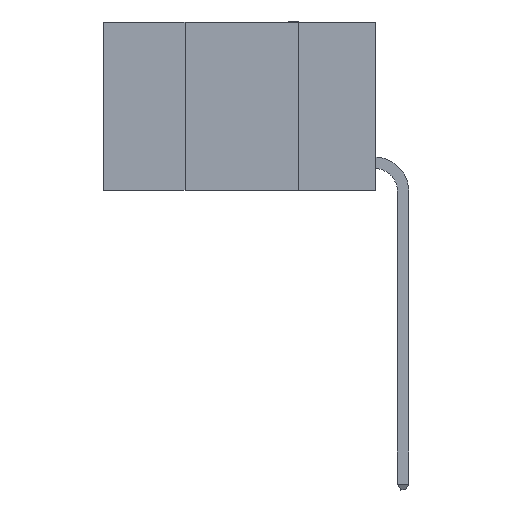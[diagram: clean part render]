
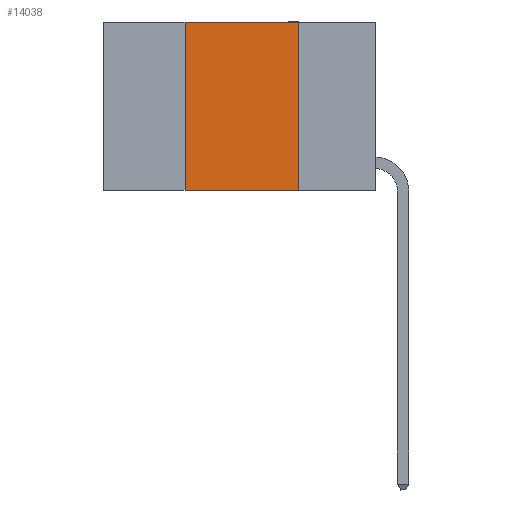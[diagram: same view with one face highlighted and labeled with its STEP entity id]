
A CAD part, left-side view. The second image highlights one B-rep face of the part: STEP entity #14038.
In plain terms, the highlighted planar face has unit normal (-1, 0, 0).
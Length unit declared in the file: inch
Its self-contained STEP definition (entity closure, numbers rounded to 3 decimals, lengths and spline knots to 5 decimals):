
#351 = EDGE_LOOP ( 'NONE', ( #9684, #9820, #11983, #7212 ) ) ;
#1173 = DIRECTION ( 'NONE',  ( 0., 0., 1. ) ) ;
#1195 = CARTESIAN_POINT ( 'NONE',  ( 0., 0.17, 0. ) ) ;
#1365 = VERTEX_POINT ( 'NONE', #11477 ) ;
#1875 = LINE ( 'NONE', #8475, #10111 ) ;
#2603 = DIRECTION ( 'NONE',  ( 0., -1., 0. ) ) ;
#2789 = PLANE ( 'NONE',  #8046 ) ;
#3417 = EDGE_CURVE ( 'NONE', #16266, #13395, #12868, .T. ) ;
#3720 = VECTOR ( 'NONE', #2603, 39.37008 ) ;
#3760 = VERTEX_POINT ( 'NONE', #4488 ) ;
#4374 = EDGE_CURVE ( 'NONE', #13395, #3760, #1875, .T. ) ;
#4488 = CARTESIAN_POINT ( 'NONE',  ( 0., 0.17, 0. ) ) ;
#5959 = FACE_OUTER_BOUND ( 'NONE', #351, .T. ) ;
#7212 = ORIENTED_EDGE ( 'NONE', *, *, #7569, .T. ) ;
#7569 = EDGE_CURVE ( 'NONE', #16266, #1365, #10730, .T. ) ;
#8046 = AXIS2_PLACEMENT_3D ( 'NONE', #17712, #12679, #11143 ) ;
#8475 = CARTESIAN_POINT ( 'NONE',  ( 0., 0.6, 0. ) ) ;
#9258 = EDGE_CURVE ( 'NONE', #3760, #1365, #17725, .T. ) ;
#9475 = VECTOR ( 'NONE', #14088, 39.37008 ) ;
#9684 = ORIENTED_EDGE ( 'NONE', *, *, #9258, .F. ) ;
#9820 = ORIENTED_EDGE ( 'NONE', *, *, #4374, .F. ) ;
#9994 = DIRECTION ( 'NONE',  ( 0., -1., 0. ) ) ;
#10111 = VECTOR ( 'NONE', #9994, 39.37008 ) ;
#10730 = LINE ( 'NONE', #15791, #3720 ) ;
#11143 = DIRECTION ( 'NONE',  ( 0., 0., -1. ) ) ;
#11477 = CARTESIAN_POINT ( 'NONE',  ( 0., 0.17, -0.37 ) ) ;
#11502 = VECTOR ( 'NONE', #1173, 39.37008 ) ;
#11569 = CARTESIAN_POINT ( 'NONE',  ( 0., 0.42, 0. ) ) ;
#11983 = ORIENTED_EDGE ( 'NONE', *, *, #3417, .F. ) ;
#12679 = DIRECTION ( 'NONE',  ( 1., 0., 0. ) ) ;
#12868 = LINE ( 'NONE', #14688, #11502 ) ;
#13395 = VERTEX_POINT ( 'NONE', #11569 ) ;
#14038 = ADVANCED_FACE ( 'NONE', ( #5959 ), #2789, .F. ) ;
#14088 = DIRECTION ( 'NONE',  ( 0., 0., -1. ) ) ;
#14443 = CARTESIAN_POINT ( 'NONE',  ( 0., 0.42, -0.37 ) ) ;
#14688 = CARTESIAN_POINT ( 'NONE',  ( 0., 0.42, 0. ) ) ;
#15791 = CARTESIAN_POINT ( 'NONE',  ( 0., 0.6, -0.37 ) ) ;
#16266 = VERTEX_POINT ( 'NONE', #14443 ) ;
#17712 = CARTESIAN_POINT ( 'NONE',  ( 0., 0.6, 0. ) ) ;
#17725 = LINE ( 'NONE', #1195, #9475 ) ;
